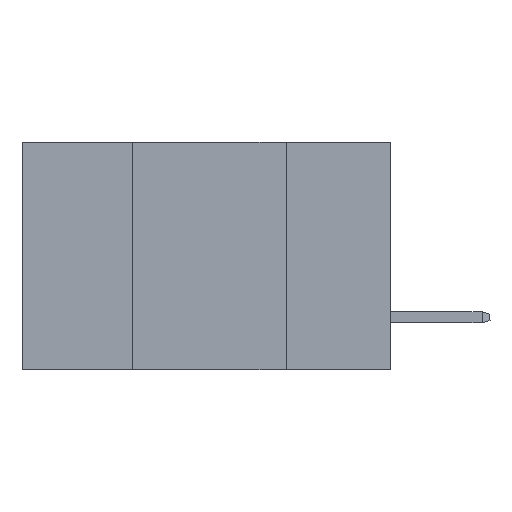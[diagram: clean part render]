
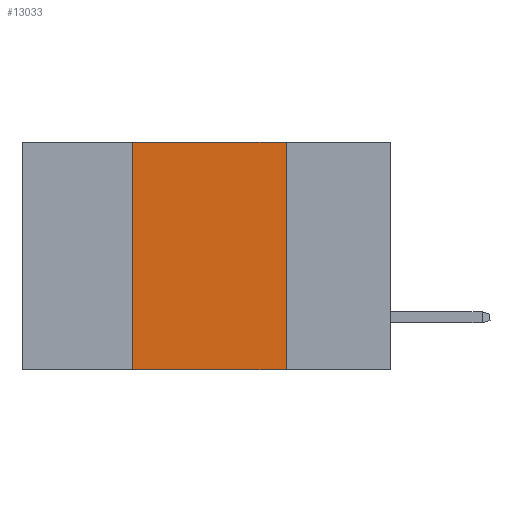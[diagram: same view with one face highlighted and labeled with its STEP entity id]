
A CAD part, left-side view. The second image highlights one B-rep face of the part: STEP entity #13033.
In plain terms, the highlighted planar face has unit normal (-1, 0, 0).
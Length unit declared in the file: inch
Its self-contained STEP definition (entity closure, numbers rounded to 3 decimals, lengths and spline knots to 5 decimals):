
#706 = DIRECTION ( 'NONE',  ( 0., -1., 0. ) ) ;
#914 = LINE ( 'NONE', #8711, #20872 ) ;
#1242 = VERTEX_POINT ( 'NONE', #22255 ) ;
#1290 = ORIENTED_EDGE ( 'NONE', *, *, #18557, .T. ) ;
#1792 = VERTEX_POINT ( 'NONE', #7993 ) ;
#3064 = VERTEX_POINT ( 'NONE', #18146 ) ;
#3193 = CARTESIAN_POINT ( 'NONE',  ( 0., 0.42, 0. ) ) ;
#5195 = CARTESIAN_POINT ( 'NONE',  ( 0., 0.17, 0. ) ) ;
#5794 = VECTOR ( 'NONE', #706, 39.37008 ) ;
#6302 = AXIS2_PLACEMENT_3D ( 'NONE', #12291, #6471, #19869 ) ;
#6471 = DIRECTION ( 'NONE',  ( 1., 0., 0. ) ) ;
#6724 = VERTEX_POINT ( 'NONE', #25010 ) ;
#7593 = EDGE_CURVE ( 'NONE', #3064, #6724, #21062, .T. ) ;
#7751 = EDGE_CURVE ( 'NONE', #1242, #3064, #7975, .T. ) ;
#7975 = LINE ( 'NONE', #3193, #17522 ) ;
#7993 = CARTESIAN_POINT ( 'NONE',  ( 0., 0.17, -0.37 ) ) ;
#8711 = CARTESIAN_POINT ( 'NONE',  ( 0., 0.6, -0.37 ) ) ;
#10015 = ORIENTED_EDGE ( 'NONE', *, *, #7593, .F. ) ;
#10662 = DIRECTION ( 'NONE',  ( 0., -1., 0. ) ) ;
#11219 = ORIENTED_EDGE ( 'NONE', *, *, #7751, .F. ) ;
#12291 = CARTESIAN_POINT ( 'NONE',  ( 0., 0.6, 0. ) ) ;
#12640 = EDGE_CURVE ( 'NONE', #6724, #1792, #24666, .T. ) ;
#13033 = ADVANCED_FACE ( 'NONE', ( #22025 ), #17974, .F. ) ;
#16774 = DIRECTION ( 'NONE',  ( 0., 0., -1. ) ) ;
#17522 = VECTOR ( 'NONE', #18642, 39.37008 ) ;
#17974 = PLANE ( 'NONE',  #6302 ) ;
#18146 = CARTESIAN_POINT ( 'NONE',  ( 0., 0.42, 0. ) ) ;
#18557 = EDGE_CURVE ( 'NONE', #1242, #1792, #914, .T. ) ;
#18642 = DIRECTION ( 'NONE',  ( 0., 0., 1. ) ) ;
#19075 = VECTOR ( 'NONE', #16774, 39.37008 ) ;
#19869 = DIRECTION ( 'NONE',  ( 0., 0., -1. ) ) ;
#20037 = EDGE_LOOP ( 'NONE', ( #24473, #10015, #11219, #1290 ) ) ;
#20872 = VECTOR ( 'NONE', #10662, 39.37008 ) ;
#21062 = LINE ( 'NONE', #23823, #5794 ) ;
#22025 = FACE_OUTER_BOUND ( 'NONE', #20037, .T. ) ;
#22255 = CARTESIAN_POINT ( 'NONE',  ( 0., 0.42, -0.37 ) ) ;
#23823 = CARTESIAN_POINT ( 'NONE',  ( 0., 0.6, 0. ) ) ;
#24473 = ORIENTED_EDGE ( 'NONE', *, *, #12640, .F. ) ;
#24666 = LINE ( 'NONE', #5195, #19075 ) ;
#25010 = CARTESIAN_POINT ( 'NONE',  ( 0., 0.17, 0. ) ) ;
